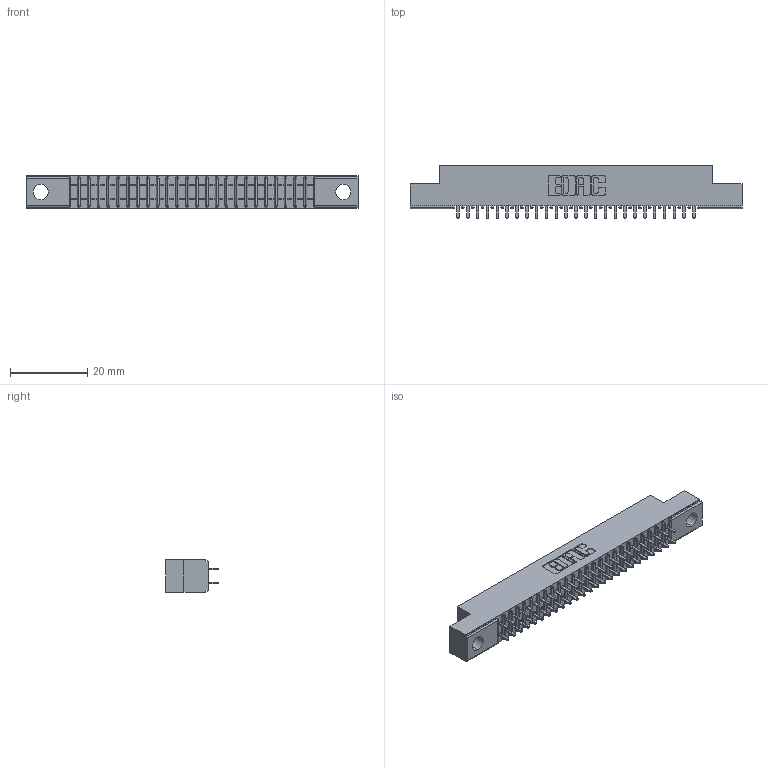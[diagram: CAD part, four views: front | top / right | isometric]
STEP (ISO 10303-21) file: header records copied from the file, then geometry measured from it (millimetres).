
FILE_DESCRIPTION (( 'STEP AP203' ), '1' );
FILE_NAME ('391-050-524-204.STEP', '2018-08-09T05:17:57', ( '' ), ( '' ), 'SwSTEP 2.0', 'SolidWorks 2016', '' );
FILE_SCHEMA (( 'CONFIG_CONTROL_DESIGN' ));
Length unit declared in the file: inch
Products named in the file (3): 391-050-524-204; 341 Part_.156 (3.96) Dia Mounting Holes; 341-292-001_341-292-124
Assembly tree (51 placements, depth 2):
  391-050-524-204
    341 Part_.156 (3.96) Dia Mounting Holes
    341-292-001_341-292-124  x50
Bounding box: 85.72 x 13.64 x 8.38 mm (x, y, z)
Volume: 4761.6 mm3; surface area: 9925.9 mm2
Topology: 51 solids, 51 shells, 3430 faces, 9927 edges, 6430 vertices
Faces by surface type: plane 2082, cylinder 1248, sphere 52, torus 48
Entity records: 32938 total; most frequent: CARTESIAN_POINT 5481, ORIENTED_EDGE 5442, DIRECTION 5323, EDGE_CURVE 2721, LINE 2187, VECTOR 2187, VERTEX_POINT 1726, AXIS2_PLACEMENT_3D 1568
